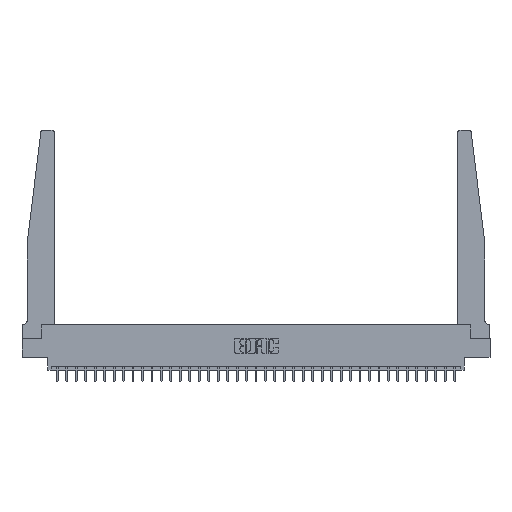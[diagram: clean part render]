
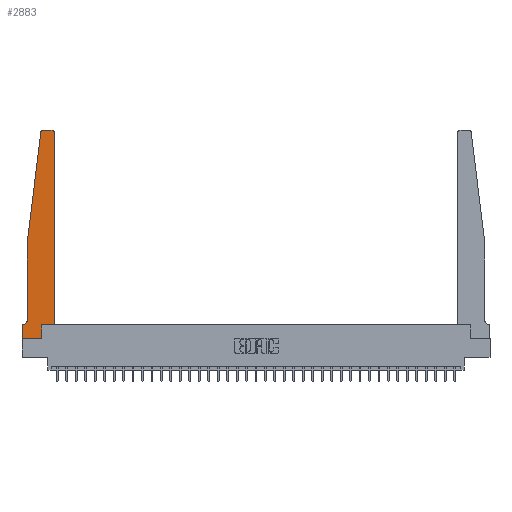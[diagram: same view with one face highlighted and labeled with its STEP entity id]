
A CAD part, top view. The second image highlights one B-rep face of the part: STEP entity #2883.
In plain terms, the highlighted planar face has unit normal (0, 0, 1).
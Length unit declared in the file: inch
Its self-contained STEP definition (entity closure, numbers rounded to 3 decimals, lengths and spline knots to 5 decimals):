
#183 = CARTESIAN_POINT ( 'NONE',  ( 0.015, 0.2375, 0.37 ) ) ;
#412 = ORIENTED_EDGE ( 'NONE', *, *, #6423, .T. ) ;
#660 = ORIENTED_EDGE ( 'NONE', *, *, #28956, .T. ) ;
#724 = CARTESIAN_POINT ( 'NONE',  ( 0., 0., 0.37 ) ) ;
#834 = CARTESIAN_POINT ( 'NONE',  ( 0.015, 0.1875, 0.37 ) ) ;
#1696 = CARTESIAN_POINT ( 'NONE',  ( 0.27653, 2.75, 0.37 ) ) ;
#1827 = CARTESIAN_POINT ( 'NONE',  ( 0.27653, 2.72, 0.37 ) ) ;
#2658 = CARTESIAN_POINT ( 'NONE',  ( 0., 0., 0.37 ) ) ;
#2883 = ADVANCED_FACE ( 'NONE', ( #30543 ), #12385, .T. ) ;
#2918 = DIRECTION ( 'NONE',  ( 1., 0., 0. ) ) ;
#2946 = CARTESIAN_POINT ( 'NONE',  ( 0.2605, 0., 0.37 ) ) ;
#3485 = ORIENTED_EDGE ( 'NONE', *, *, #16987, .T. ) ;
#3647 = VERTEX_POINT ( 'NONE', #8894 ) ;
#4423 = EDGE_CURVE ( 'NONE', #13678, #3647, #31396, .T. ) ;
#4484 = ORIENTED_EDGE ( 'NONE', *, *, #11574, .T. ) ;
#4634 = DIRECTION ( 'NONE',  ( -1., 0., 0. ) ) ;
#5584 = CARTESIAN_POINT ( 'NONE',  ( 0.395, 2.72, 0.37 ) ) ;
#5607 = ORIENTED_EDGE ( 'NONE', *, *, #21989, .T. ) ;
#5931 = VECTOR ( 'NONE', #4634, 39.37008 ) ;
#6423 = EDGE_CURVE ( 'NONE', #13249, #23721, #7699, .T. ) ;
#6764 = DIRECTION ( 'NONE',  ( 1., 0., 0. ) ) ;
#7012 = CARTESIAN_POINT ( 'NONE',  ( 0.065, 1.25, 0.37 ) ) ;
#7176 = DIRECTION ( 'NONE',  ( 0., -1., 0. ) ) ;
#7466 = CARTESIAN_POINT ( 'NONE',  ( 0., 0.1875, 0.37 ) ) ;
#7525 = CIRCLE ( 'NONE', #31766, 0.05 ) ;
#7699 = LINE ( 'NONE', #17995, #13684 ) ;
#7824 = VECTOR ( 'NONE', #24051, 39.37008 ) ;
#7991 = EDGE_CURVE ( 'NONE', #3647, #20480, #29140, .T. ) ;
#8528 = VERTEX_POINT ( 'NONE', #20440 ) ;
#8894 = CARTESIAN_POINT ( 'NONE',  ( 0.425, 0.18, 0.37 ) ) ;
#9385 = LINE ( 'NONE', #7012, #16675 ) ;
#9471 = ORIENTED_EDGE ( 'NONE', *, *, #24484, .T. ) ;
#9510 = CARTESIAN_POINT ( 'NONE',  ( 0.425, 2.72, 0.37 ) ) ;
#9762 = DIRECTION ( 'NONE',  ( -1., 0., 0. ) ) ;
#10031 = VECTOR ( 'NONE', #27616, 39.37008 ) ;
#10242 = VECTOR ( 'NONE', #6764, 39.37008 ) ;
#10477 = DIRECTION ( 'NONE',  ( 1., 0., 0. ) ) ;
#10490 = EDGE_CURVE ( 'NONE', #16751, #33208, #30775, .T. ) ;
#11169 = VERTEX_POINT ( 'NONE', #32579 ) ;
#11574 = EDGE_CURVE ( 'NONE', #26206, #13678, #27466, .T. ) ;
#11957 = CARTESIAN_POINT ( 'NONE',  ( 0., 0., 0.37 ) ) ;
#12385 = PLANE ( 'NONE',  #24405 ) ;
#12857 = CARTESIAN_POINT ( 'NONE',  ( 0., 0.1875, 0.37 ) ) ;
#13019 = VERTEX_POINT ( 'NONE', #1696 ) ;
#13249 = VERTEX_POINT ( 'NONE', #834 ) ;
#13403 = VERTEX_POINT ( 'NONE', #11957 ) ;
#13554 = LINE ( 'NONE', #724, #10242 ) ;
#13678 = VERTEX_POINT ( 'NONE', #28927 ) ;
#13684 = VECTOR ( 'NONE', #9762, 39.37008 ) ;
#13821 = DIRECTION ( 'NONE',  ( 0., 0., 1. ) ) ;
#15127 = EDGE_LOOP ( 'NONE', ( #22269, #3485, #20898, #5607, #18877, #412, #660, #9471, #4484, #19329, #23931, #16177 ) ) ;
#15195 = DIRECTION ( 'NONE',  ( 0., 0., -1. ) ) ;
#15533 = EDGE_CURVE ( 'NONE', #20480, #8528, #29522, .T. ) ;
#16177 = ORIENTED_EDGE ( 'NONE', *, *, #15533, .T. ) ;
#16675 = VECTOR ( 'NONE', #7176, 39.37008 ) ;
#16748 = EDGE_CURVE ( 'NONE', #11169, #13249, #7525, .T. ) ;
#16751 = VERTEX_POINT ( 'NONE', #25441 ) ;
#16812 = DIRECTION ( 'NONE',  ( 0., -1., 0. ) ) ;
#16854 = DIRECTION ( 'NONE',  ( 0., 0., 1. ) ) ;
#16987 = EDGE_CURVE ( 'NONE', #13019, #16751, #25286, .T. ) ;
#17995 = CARTESIAN_POINT ( 'NONE',  ( 0.065, 0.1875, 0.37 ) ) ;
#18265 = CARTESIAN_POINT ( 'NONE',  ( 0.425, 0.18, 0.37 ) ) ;
#18877 = ORIENTED_EDGE ( 'NONE', *, *, #16748, .T. ) ;
#19016 = VECTOR ( 'NONE', #16812, 39.37008 ) ;
#19329 = ORIENTED_EDGE ( 'NONE', *, *, #4423, .T. ) ;
#20440 = CARTESIAN_POINT ( 'NONE',  ( 0.395, 2.75, 0.37 ) ) ;
#20480 = VERTEX_POINT ( 'NONE', #9510 ) ;
#20601 = LINE ( 'NONE', #30722, #5931 ) ;
#20898 = ORIENTED_EDGE ( 'NONE', *, *, #10490, .T. ) ;
#21854 = VECTOR ( 'NONE', #2918, 39.37008 ) ;
#21989 = EDGE_CURVE ( 'NONE', #33208, #11169, #9385, .T. ) ;
#22078 = CARTESIAN_POINT ( 'NONE',  ( 0.2605, 0.18, 0.37 ) ) ;
#22269 = ORIENTED_EDGE ( 'NONE', *, *, #24257, .T. ) ;
#23498 = CARTESIAN_POINT ( 'NONE',  ( 0.065, 1.25, 0.37 ) ) ;
#23721 = VERTEX_POINT ( 'NONE', #12857 ) ;
#23931 = ORIENTED_EDGE ( 'NONE', *, *, #7991, .T. ) ;
#24051 = DIRECTION ( 'NONE',  ( 0., 1., 0. ) ) ;
#24257 = EDGE_CURVE ( 'NONE', #8528, #13019, #20601, .T. ) ;
#24405 = AXIS2_PLACEMENT_3D ( 'NONE', #7466, #27338, #24811 ) ;
#24436 = CARTESIAN_POINT ( 'NONE',  ( 0.065, 1.25, 0.37 ) ) ;
#24484 = EDGE_CURVE ( 'NONE', #13403, #26206, #13554, .T. ) ;
#24751 = AXIS2_PLACEMENT_3D ( 'NONE', #1827, #16854, #27265 ) ;
#24811 = DIRECTION ( 'NONE',  ( 1., 0., 0. ) ) ;
#25286 = CIRCLE ( 'NONE', #24751, 0.03 ) ;
#25441 = CARTESIAN_POINT ( 'NONE',  ( 0.24675, 2.72367, 0.37 ) ) ;
#25715 = LINE ( 'NONE', #2658, #19016 ) ;
#26206 = VERTEX_POINT ( 'NONE', #2946 ) ;
#26599 = CARTESIAN_POINT ( 'NONE',  ( 0.425, 0.18, 0.37 ) ) ;
#27257 = VECTOR ( 'NONE', #32541, 39.37008 ) ;
#27265 = DIRECTION ( 'NONE',  ( 1., 0., 0. ) ) ;
#27338 = DIRECTION ( 'NONE',  ( 0., 0., 1. ) ) ;
#27466 = LINE ( 'NONE', #22078, #27257 ) ;
#27616 = DIRECTION ( 'NONE',  ( -0.122, -0.992, 0. ) ) ;
#28927 = CARTESIAN_POINT ( 'NONE',  ( 0.2605, 0.18, 0.37 ) ) ;
#28956 = EDGE_CURVE ( 'NONE', #23721, #13403, #25715, .T. ) ;
#29140 = LINE ( 'NONE', #26599, #7824 ) ;
#29522 = CIRCLE ( 'NONE', #31157, 0.03 ) ;
#30543 = FACE_OUTER_BOUND ( 'NONE', #15127, .T. ) ;
#30679 = DIRECTION ( 'NONE',  ( -1., 0., 0. ) ) ;
#30722 = CARTESIAN_POINT ( 'NONE',  ( 0.25, 2.75, 0.37 ) ) ;
#30775 = LINE ( 'NONE', #23498, #10031 ) ;
#31157 = AXIS2_PLACEMENT_3D ( 'NONE', #5584, #13821, #10477 ) ;
#31396 = LINE ( 'NONE', #18265, #21854 ) ;
#31766 = AXIS2_PLACEMENT_3D ( 'NONE', #183, #15195, #30679 ) ;
#32541 = DIRECTION ( 'NONE',  ( 0., 1., 0. ) ) ;
#32579 = CARTESIAN_POINT ( 'NONE',  ( 0.065, 0.2375, 0.37 ) ) ;
#33208 = VERTEX_POINT ( 'NONE', #24436 ) ;
